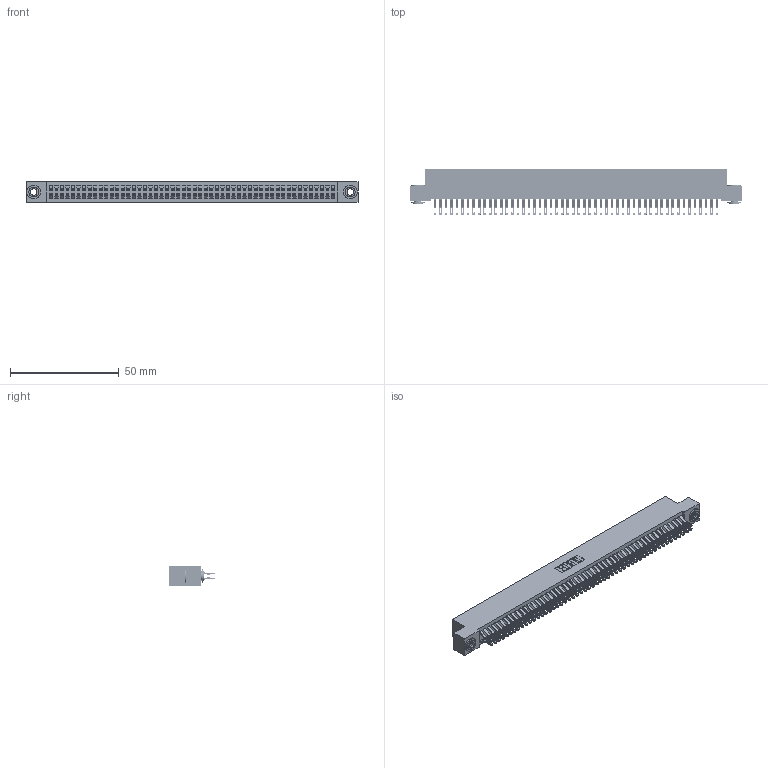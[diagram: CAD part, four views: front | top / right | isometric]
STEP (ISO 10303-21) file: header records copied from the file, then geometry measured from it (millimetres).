
FILE_DESCRIPTION (( 'STEP AP203' ), '1' );
FILE_NAME ('342-104-555-203.STEP', '2018-08-14T06:20:24', ( '' ), ( '' ), 'SwSTEP 2.0', 'SolidWorks 2016', '' );
FILE_SCHEMA (( 'CONFIG_CONTROL_DESIGN' ));
Length unit declared in the file: inch
Products named in the file (4): 342 Part_.156 TH; 345-292-001_555 Tail; 342-250-002_345-250-002-102; 342-104-555-203
Assembly tree (107 placements, depth 2):
  342-104-555-203
    342 Part_.156 TH
    345-292-001_555 Tail  x104
    342-250-002_345-250-002-102  x2
Bounding box: 152.4 x 21.47 x 9.4 mm (x, y, z)
Volume: 14052.3 mm3; surface area: 24340.4 mm2
Topology: 107 solids, 107 shells, 6180 faces, 19407 edges, 12934 vertices
Faces by surface type: plane 3612, cylinder 2560, cone 8
Entity records: 33004 total; most frequent: CARTESIAN_POINT 5467, ORIENTED_EDGE 5366, DIRECTION 4657, EDGE_CURVE 2683, LINE 2511, VECTOR 2511, VERTEX_POINT 1786, AXIS2_PLACEMENT_3D 1073
